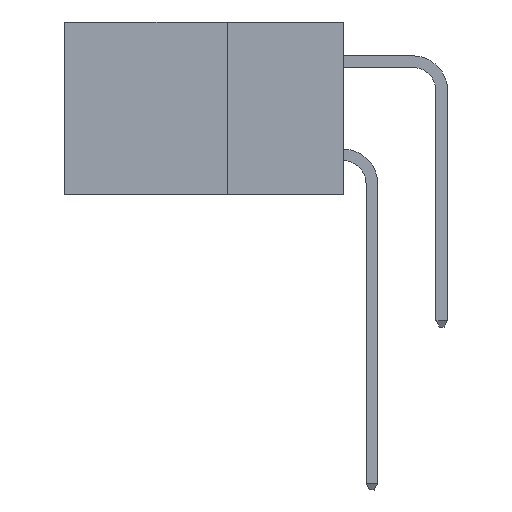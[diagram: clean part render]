
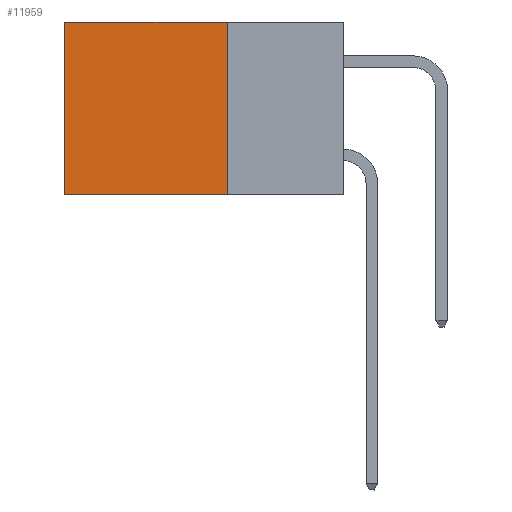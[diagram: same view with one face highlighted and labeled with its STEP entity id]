
A CAD part, left-side view. The second image highlights one B-rep face of the part: STEP entity #11959.
In plain terms, the highlighted planar face has unit normal (-1, 0, 0).
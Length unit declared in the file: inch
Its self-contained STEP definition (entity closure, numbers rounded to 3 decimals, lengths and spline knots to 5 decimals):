
#419 = CARTESIAN_POINT ( 'NONE',  ( 0.298, 0.6, -0.37 ) ) ;
#1288 = EDGE_CURVE ( 'NONE', #7199, #19082, #7195, .T. ) ;
#1749 = DIRECTION ( 'NONE',  ( 0., 0., -1. ) ) ;
#2129 = EDGE_LOOP ( 'NONE', ( #3466, #11088, #11787, #8690 ) ) ;
#2453 = LINE ( 'NONE', #8820, #17030 ) ;
#3466 = ORIENTED_EDGE ( 'NONE', *, *, #13763, .T. ) ;
#4233 = CARTESIAN_POINT ( 'NONE',  ( 0.298, 0.25, 0. ) ) ;
#4309 = DIRECTION ( 'NONE',  ( 0., 0., -1. ) ) ;
#6232 = VECTOR ( 'NONE', #11757, 39.37008 ) ;
#7195 = LINE ( 'NONE', #14743, #11890 ) ;
#7199 = VERTEX_POINT ( 'NONE', #9881 ) ;
#7667 = CARTESIAN_POINT ( 'NONE',  ( 0.298, 0.25, -0.37 ) ) ;
#7920 = DIRECTION ( 'NONE',  ( 0., 1., 0. ) ) ;
#8690 = ORIENTED_EDGE ( 'NONE', *, *, #10393, .T. ) ;
#8762 = FACE_OUTER_BOUND ( 'NONE', #2129, .T. ) ;
#8820 = CARTESIAN_POINT ( 'NONE',  ( 0.298, 0.25, -0.37 ) ) ;
#9230 = CARTESIAN_POINT ( 'NONE',  ( 0.298, 0.25, 0. ) ) ;
#9439 = DIRECTION ( 'NONE',  ( 1., 0., 0. ) ) ;
#9643 = VERTEX_POINT ( 'NONE', #13232 ) ;
#9881 = CARTESIAN_POINT ( 'NONE',  ( 0.298, 0.25, 0. ) ) ;
#10393 = EDGE_CURVE ( 'NONE', #7199, #9643, #14472, .T. ) ;
#11088 = ORIENTED_EDGE ( 'NONE', *, *, #11636, .F. ) ;
#11114 = VERTEX_POINT ( 'NONE', #419 ) ;
#11636 = EDGE_CURVE ( 'NONE', #19082, #11114, #2453, .T. ) ;
#11757 = DIRECTION ( 'NONE',  ( 0., 1., 0. ) ) ;
#11787 = ORIENTED_EDGE ( 'NONE', *, *, #1288, .F. ) ;
#11890 = VECTOR ( 'NONE', #4309, 39.37008 ) ;
#11959 = ADVANCED_FACE ( 'NONE', ( #8762 ), #16801, .F. ) ;
#12863 = DIRECTION ( 'NONE',  ( 0., 0., -1. ) ) ;
#13232 = CARTESIAN_POINT ( 'NONE',  ( 0.298, 0.6, 0. ) ) ;
#13763 = EDGE_CURVE ( 'NONE', #9643, #11114, #13799, .T. ) ;
#13799 = LINE ( 'NONE', #18798, #17629 ) ;
#14472 = LINE ( 'NONE', #4233, #6232 ) ;
#14644 = AXIS2_PLACEMENT_3D ( 'NONE', #9230, #9439, #1749 ) ;
#14743 = CARTESIAN_POINT ( 'NONE',  ( 0.298, 0.25, 0. ) ) ;
#16801 = PLANE ( 'NONE',  #14644 ) ;
#17030 = VECTOR ( 'NONE', #7920, 39.37008 ) ;
#17629 = VECTOR ( 'NONE', #12863, 39.37008 ) ;
#18798 = CARTESIAN_POINT ( 'NONE',  ( 0.298, 0.6, 0. ) ) ;
#19082 = VERTEX_POINT ( 'NONE', #7667 ) ;
